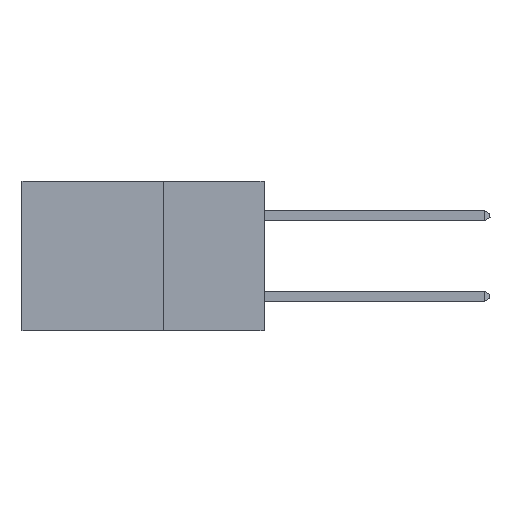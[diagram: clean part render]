
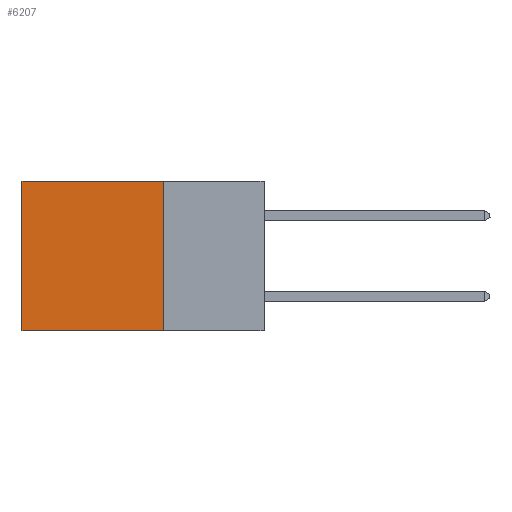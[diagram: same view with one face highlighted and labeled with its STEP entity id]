
A CAD part, left-side view. The second image highlights one B-rep face of the part: STEP entity #6207.
In plain terms, the highlighted planar face has unit normal (-1, 0, 0).
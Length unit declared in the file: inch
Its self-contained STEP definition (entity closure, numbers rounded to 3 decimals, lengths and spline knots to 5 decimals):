
#514 = ORIENTED_EDGE ( 'NONE', *, *, #1711, .T. ) ;
#1406 = CARTESIAN_POINT ( 'NONE',  ( 0.298, 0.25, 0. ) ) ;
#1711 = EDGE_CURVE ( 'NONE', #17088, #21120, #18421, .T. ) ;
#2993 = CARTESIAN_POINT ( 'NONE',  ( 0.298, 0.25, 0. ) ) ;
#2999 = CARTESIAN_POINT ( 'NONE',  ( 0.298, 0.25, 0. ) ) ;
#3734 = LINE ( 'NONE', #14312, #19158 ) ;
#3782 = VECTOR ( 'NONE', #11224, 39.37008 ) ;
#3993 = ORIENTED_EDGE ( 'NONE', *, *, #6267, .F. ) ;
#4247 = DIRECTION ( 'NONE',  ( 0., 1., 0. ) ) ;
#5058 = DIRECTION ( 'NONE',  ( 1., 0., 0. ) ) ;
#5571 = DIRECTION ( 'NONE',  ( 0., 1., 0. ) ) ;
#6207 = ADVANCED_FACE ( 'NONE', ( #15799 ), #17108, .F. ) ;
#6213 = ORIENTED_EDGE ( 'NONE', *, *, #21704, .T. ) ;
#6267 = EDGE_CURVE ( 'NONE', #10215, #21094, #19859, .T. ) ;
#9199 = CARTESIAN_POINT ( 'NONE',  ( 0.298, 0.25, 0. ) ) ;
#9211 = LINE ( 'NONE', #1406, #24485 ) ;
#10215 = VERTEX_POINT ( 'NONE', #2999 ) ;
#10900 = AXIS2_PLACEMENT_3D ( 'NONE', #2993, #5058, #19117 ) ;
#11224 = DIRECTION ( 'NONE',  ( 0., 0., -1. ) ) ;
#12881 = ORIENTED_EDGE ( 'NONE', *, *, #17605, .F. ) ;
#13683 = CARTESIAN_POINT ( 'NONE',  ( 0.298, 0.6, 0. ) ) ;
#14312 = CARTESIAN_POINT ( 'NONE',  ( 0.298, 0.25, -0.37 ) ) ;
#15799 = FACE_OUTER_BOUND ( 'NONE', #21932, .T. ) ;
#17088 = VERTEX_POINT ( 'NONE', #24626 ) ;
#17108 = PLANE ( 'NONE',  #10900 ) ;
#17605 = EDGE_CURVE ( 'NONE', #21094, #21120, #3734, .T. ) ;
#18421 = LINE ( 'NONE', #13683, #23063 ) ;
#19117 = DIRECTION ( 'NONE',  ( 0., 0., -1. ) ) ;
#19158 = VECTOR ( 'NONE', #4247, 39.37008 ) ;
#19745 = CARTESIAN_POINT ( 'NONE',  ( 0.298, 0.6, -0.37 ) ) ;
#19859 = LINE ( 'NONE', #9199, #3782 ) ;
#21094 = VERTEX_POINT ( 'NONE', #21648 ) ;
#21120 = VERTEX_POINT ( 'NONE', #19745 ) ;
#21648 = CARTESIAN_POINT ( 'NONE',  ( 0.298, 0.25, -0.37 ) ) ;
#21704 = EDGE_CURVE ( 'NONE', #10215, #17088, #9211, .T. ) ;
#21932 = EDGE_LOOP ( 'NONE', ( #514, #12881, #3993, #6213 ) ) ;
#23063 = VECTOR ( 'NONE', #24808, 39.37008 ) ;
#24485 = VECTOR ( 'NONE', #5571, 39.37008 ) ;
#24626 = CARTESIAN_POINT ( 'NONE',  ( 0.298, 0.6, 0. ) ) ;
#24808 = DIRECTION ( 'NONE',  ( 0., 0., -1. ) ) ;
